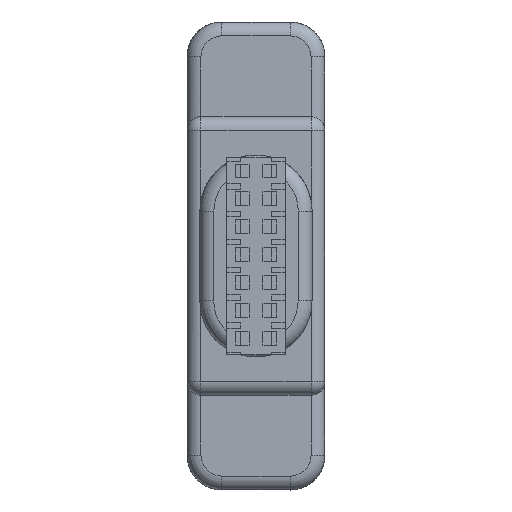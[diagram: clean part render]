
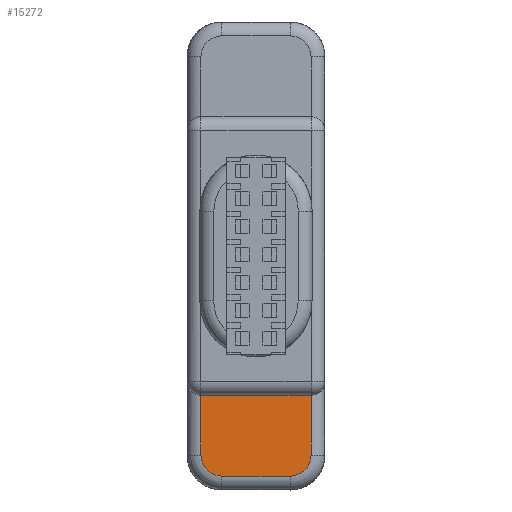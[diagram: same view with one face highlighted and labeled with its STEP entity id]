
A CAD part, left-side view. The second image highlights one B-rep face of the part: STEP entity #15272.
In plain terms, the highlighted planar face has unit normal (-1, 0, 0).
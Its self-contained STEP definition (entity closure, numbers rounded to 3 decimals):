
#719 = VERTEX_POINT ( 'NONE', #9767 ) ;
#721 = PLANE ( 'NONE',  #34426 ) ;
#1794 = CARTESIAN_POINT ( 'NONE',  ( -129.673, -4.162, -15.495 ) ) ;
#2005 = CARTESIAN_POINT ( 'NONE',  ( -129.673, -11.484, -14.492 ) ) ;
#2191 = CARTESIAN_POINT ( 'NONE',  ( -129.673, -6.217, -9.995 ) ) ;
#2848 = CARTESIAN_POINT ( 'NONE',  ( -129.673, -5.084, -15.795 ) ) ;
#3080 = B_SPLINE_CURVE_WITH_KNOTS ( 'NONE', 3,
 ( #12531, #14816, #23110, #25213, #1794, #30846, #17486, #19922, #31365, #31011 ),
 .UNSPECIFIED., .F., .F.,
 ( 4, 2, 2, 2, 4 ),
 ( 0., 0.25, 0.5, 0.75, 1. ),
 .UNSPECIFIED. ) ;
#4799 = CARTESIAN_POINT ( 'NONE',  ( -129.673, -11.484, -11.429 ) ) ;
#5740 = CARTESIAN_POINT ( 'NONE',  ( -129.673, -6.717, -15.795 ) ) ;
#5767 = VERTEX_POINT ( 'NONE', #16958 ) ;
#6171 = DIRECTION ( 'NONE',  ( 0., 1., 0. ) ) ;
#6960 = CARTESIAN_POINT ( 'NONE',  ( -129.673, -11.445, -14.688 ) ) ;
#7936 = B_SPLINE_CURVE_WITH_KNOTS ( 'NONE', 3,
 ( #30975, #31509, #9867, #12666 ),
 .UNSPECIFIED., .F., .F.,
 ( 4, 4 ),
 ( 0., 1. ),
 .UNSPECIFIED. ) ;
#8204 = CARTESIAN_POINT ( 'NONE',  ( -129.673, -9.984, -15.795 ) ) ;
#9767 = CARTESIAN_POINT ( 'NONE',  ( -129.673, -11.484, -9.996 ) ) ;
#9867 = CARTESIAN_POINT ( 'NONE',  ( -129.673, -3.584, -11.428 ) ) ;
#9949 = CARTESIAN_POINT ( 'NONE',  ( -129.673, -10.739, -15.606 ) ) ;
#10657 = CARTESIAN_POINT ( 'NONE',  ( -129.673, -8.851, -9.995 ) ) ;
#11151 = CARTESIAN_POINT ( 'NONE',  ( -129.673, -9.984, -15.795 ) ) ;
#11555 = CARTESIAN_POINT ( 'NONE',  ( -129.673, -8.35, -15.795 ) ) ;
#11710 = EDGE_CURVE ( 'NONE', #719, #5767, #17746, .T. ) ;
#12531 = CARTESIAN_POINT ( 'NONE',  ( -129.673, -5.084, -15.795 ) ) ;
#12666 = CARTESIAN_POINT ( 'NONE',  ( -129.673, -3.584, -9.995 ) ) ;
#13046 = VERTEX_POINT ( 'NONE', #2848 ) ;
#13397 = DIRECTION ( 'NONE',  ( 1., 0., 0. ) ) ;
#13828 = VERTEX_POINT ( 'NONE', #32778 ) ;
#13832 = ORIENTED_EDGE ( 'NONE', *, *, #34617, .F. ) ;
#14816 = CARTESIAN_POINT ( 'NONE',  ( -129.673, -4.887, -15.795 ) ) ;
#14882 = B_SPLINE_CURVE_WITH_KNOTS ( 'NONE', 3,
 ( #22963, #2005, #6960, #25934, #22127, #33886, #9949, #32884, #30241, #26470 ),
 .UNSPECIFIED., .F., .F.,
 ( 4, 2, 2, 2, 4 ),
 ( 0., 0.25, 0.5, 0.75, 1. ),
 .UNSPECIFIED. ) ;
#15272 = ADVANCED_FACE ( 'NONE', ( #26753 ), #721, .F. ) ;
#15582 = CARTESIAN_POINT ( 'NONE',  ( -129.673, -11.484, -9.996 ) ) ;
#15671 = EDGE_CURVE ( 'NONE', #16870, #22309, #14882, .T. ) ;
#15889 = CARTESIAN_POINT ( 'NONE',  ( -129.673, -11.484, -12.862 ) ) ;
#15913 = EDGE_CURVE ( 'NONE', #13046, #13828, #3080, .T. ) ;
#16870 = VERTEX_POINT ( 'NONE', #28326 ) ;
#16958 = CARTESIAN_POINT ( 'NONE',  ( -129.673, -3.584, -9.995 ) ) ;
#17486 = CARTESIAN_POINT ( 'NONE',  ( -129.673, -3.773, -15.05 ) ) ;
#17746 = B_SPLINE_CURVE_WITH_KNOTS ( 'NONE', 3,
 ( #15582, #10657, #2191, #29944 ),
 .UNSPECIFIED., .F., .F.,
 ( 4, 4 ),
 ( 0., 1. ),
 .UNSPECIFIED. ) ;
#17805 = EDGE_LOOP ( 'NONE', ( #24904, #13832, #24331, #34242, #23415, #18090 ) ) ;
#18090 = ORIENTED_EDGE ( 'NONE', *, *, #19988, .F. ) ;
#19922 = CARTESIAN_POINT ( 'NONE',  ( -129.673, -3.623, -14.688 ) ) ;
#19988 = EDGE_CURVE ( 'NONE', #13828, #5767, #7936, .T. ) ;
#21648 = CARTESIAN_POINT ( 'NONE',  ( -129.673, -7.534, -12.895 ) ) ;
#21682 = B_SPLINE_CURVE_WITH_KNOTS ( 'NONE', 3,
 ( #34214, #4799, #15889, #31743 ),
 .UNSPECIFIED., .F., .F.,
 ( 4, 4 ),
 ( 0., 1. ),
 .UNSPECIFIED. ) ;
#22127 = CARTESIAN_POINT ( 'NONE',  ( -129.673, -11.183, -15.217 ) ) ;
#22309 = VERTEX_POINT ( 'NONE', #11151 ) ;
#22963 = CARTESIAN_POINT ( 'NONE',  ( -129.673, -11.484, -14.296 ) ) ;
#23110 = CARTESIAN_POINT ( 'NONE',  ( -129.673, -4.691, -15.756 ) ) ;
#23415 = ORIENTED_EDGE ( 'NONE', *, *, #11710, .T. ) ;
#24331 = ORIENTED_EDGE ( 'NONE', *, *, #15671, .F. ) ;
#24590 = CARTESIAN_POINT ( 'NONE',  ( -129.673, -5.084, -15.795 ) ) ;
#24904 = ORIENTED_EDGE ( 'NONE', *, *, #15913, .F. ) ;
#25213 = CARTESIAN_POINT ( 'NONE',  ( -129.673, -4.328, -15.606 ) ) ;
#25934 = CARTESIAN_POINT ( 'NONE',  ( -129.673, -11.294, -15.051 ) ) ;
#26470 = CARTESIAN_POINT ( 'NONE',  ( -129.673, -9.984, -15.795 ) ) ;
#26753 = FACE_OUTER_BOUND ( 'NONE', #17805, .T. ) ;
#28326 = CARTESIAN_POINT ( 'NONE',  ( -129.673, -11.484, -14.296 ) ) ;
#28878 = EDGE_CURVE ( 'NONE', #719, #16870, #21682, .T. ) ;
#29944 = CARTESIAN_POINT ( 'NONE',  ( -129.673, -3.584, -9.995 ) ) ;
#30241 = CARTESIAN_POINT ( 'NONE',  ( -129.673, -10.18, -15.796 ) ) ;
#30846 = CARTESIAN_POINT ( 'NONE',  ( -129.673, -3.884, -15.217 ) ) ;
#30975 = CARTESIAN_POINT ( 'NONE',  ( -129.673, -3.584, -14.295 ) ) ;
#31011 = CARTESIAN_POINT ( 'NONE',  ( -129.673, -3.584, -14.295 ) ) ;
#31365 = CARTESIAN_POINT ( 'NONE',  ( -129.673, -3.584, -14.491 ) ) ;
#31509 = CARTESIAN_POINT ( 'NONE',  ( -129.673, -3.584, -12.862 ) ) ;
#31743 = CARTESIAN_POINT ( 'NONE',  ( -129.673, -11.484, -14.296 ) ) ;
#32778 = CARTESIAN_POINT ( 'NONE',  ( -129.673, -3.584, -14.295 ) ) ;
#32884 = CARTESIAN_POINT ( 'NONE',  ( -129.673, -10.376, -15.756 ) ) ;
#33542 = B_SPLINE_CURVE_WITH_KNOTS ( 'NONE', 3,
 ( #8204, #11555, #5740, #24590 ),
 .UNSPECIFIED., .F., .F.,
 ( 4, 4 ),
 ( 0., 1. ),
 .UNSPECIFIED. ) ;
#33886 = CARTESIAN_POINT ( 'NONE',  ( -129.673, -10.905, -15.495 ) ) ;
#34214 = CARTESIAN_POINT ( 'NONE',  ( -129.673, -11.484, -9.996 ) ) ;
#34242 = ORIENTED_EDGE ( 'NONE', *, *, #28878, .F. ) ;
#34426 = AXIS2_PLACEMENT_3D ( 'NONE', #21648, #13397, #6171 ) ;
#34617 = EDGE_CURVE ( 'NONE', #22309, #13046, #33542, .T. ) ;
